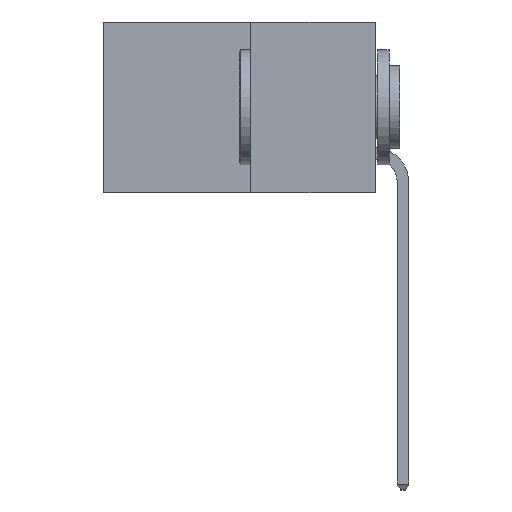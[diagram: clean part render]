
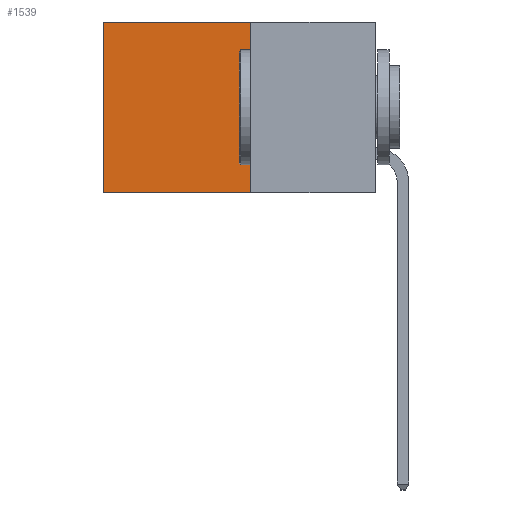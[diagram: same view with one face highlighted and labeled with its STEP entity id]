
A CAD part, left-side view. The second image highlights one B-rep face of the part: STEP entity #1539.
In plain terms, the highlighted planar face has unit normal (-1, 0, 0).
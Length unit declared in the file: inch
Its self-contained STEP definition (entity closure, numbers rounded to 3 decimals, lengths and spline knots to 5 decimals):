
#141 = DIRECTION ( 'NONE',  ( 0., 0., -1. ) ) ;
#401 = DIRECTION ( 'NONE',  ( 0., 1., 0. ) ) ;
#494 = CARTESIAN_POINT ( 'NONE',  ( 0.277, 0.27, 0. ) ) ;
#1015 = LINE ( 'NONE', #7336, #7319 ) ;
#1264 = DIRECTION ( 'NONE',  ( 0., 0., -1. ) ) ;
#1281 = CARTESIAN_POINT ( 'NONE',  ( 0.277, 0.59, -0.37 ) ) ;
#1539 = ADVANCED_FACE ( 'NONE', ( #7823 ), #5206, .F. ) ;
#1997 = CARTESIAN_POINT ( 'NONE',  ( 0.277, 0.27, -0.37 ) ) ;
#2983 = VERTEX_POINT ( 'NONE', #10351 ) ;
#4017 = DIRECTION ( 'NONE',  ( 0., 0., -1. ) ) ;
#4320 = VERTEX_POINT ( 'NONE', #7296 ) ;
#4783 = CARTESIAN_POINT ( 'NONE',  ( 0.277, 0.27, -0.37 ) ) ;
#4795 = CARTESIAN_POINT ( 'NONE',  ( 0.277, 0.27, 0. ) ) ;
#4800 = VECTOR ( 'NONE', #401, 39.37008 ) ;
#4980 = LINE ( 'NONE', #1281, #9222 ) ;
#5073 = LINE ( 'NONE', #494, #4800 ) ;
#5206 = PLANE ( 'NONE',  #7666 ) ;
#5353 = EDGE_CURVE ( 'NONE', #4320, #10902, #1015, .T. ) ;
#5619 = EDGE_CURVE ( 'NONE', #10180, #2983, #5073, .T. ) ;
#6641 = VECTOR ( 'NONE', #141, 39.37008 ) ;
#7092 = ORIENTED_EDGE ( 'NONE', *, *, #9030, .T. ) ;
#7110 = DIRECTION ( 'NONE',  ( 0., 1., 0. ) ) ;
#7296 = CARTESIAN_POINT ( 'NONE',  ( 0.277, 0.27, -0.37 ) ) ;
#7319 = VECTOR ( 'NONE', #7110, 39.37008 ) ;
#7336 = CARTESIAN_POINT ( 'NONE',  ( 0.277, 0.27, -0.37 ) ) ;
#7353 = ORIENTED_EDGE ( 'NONE', *, *, #10773, .F. ) ;
#7666 = AXIS2_PLACEMENT_3D ( 'NONE', #1997, #11151, #4017 ) ;
#7823 = FACE_OUTER_BOUND ( 'NONE', #9198, .T. ) ;
#9030 = EDGE_CURVE ( 'NONE', #2983, #10902, #4980, .T. ) ;
#9192 = CARTESIAN_POINT ( 'NONE',  ( 0.277, 0.59, -0.37 ) ) ;
#9198 = EDGE_LOOP ( 'NONE', ( #7092, #9328, #7353, #9602 ) ) ;
#9222 = VECTOR ( 'NONE', #1264, 39.37008 ) ;
#9328 = ORIENTED_EDGE ( 'NONE', *, *, #5353, .F. ) ;
#9602 = ORIENTED_EDGE ( 'NONE', *, *, #5619, .T. ) ;
#10180 = VERTEX_POINT ( 'NONE', #4795 ) ;
#10351 = CARTESIAN_POINT ( 'NONE',  ( 0.277, 0.59, 0. ) ) ;
#10773 = EDGE_CURVE ( 'NONE', #10180, #4320, #11064, .T. ) ;
#10902 = VERTEX_POINT ( 'NONE', #9192 ) ;
#11064 = LINE ( 'NONE', #4783, #6641 ) ;
#11151 = DIRECTION ( 'NONE',  ( 1., 0., 0. ) ) ;
